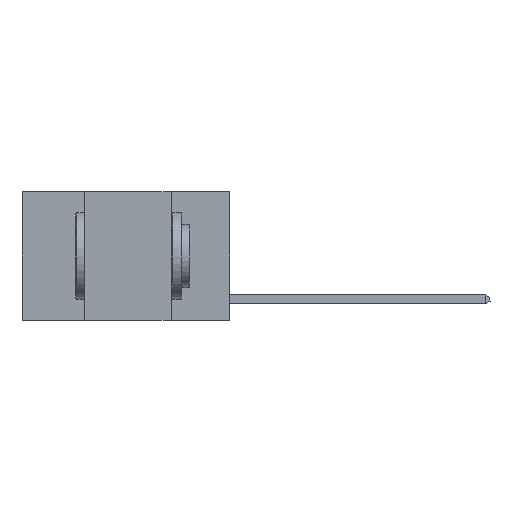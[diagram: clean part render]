
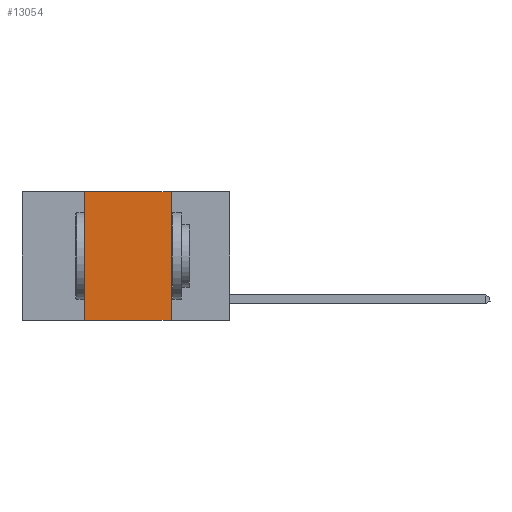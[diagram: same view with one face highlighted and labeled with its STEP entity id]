
A CAD part, left-side view. The second image highlights one B-rep face of the part: STEP entity #13054.
In plain terms, the highlighted planar face has unit normal (-1, 0, 0).
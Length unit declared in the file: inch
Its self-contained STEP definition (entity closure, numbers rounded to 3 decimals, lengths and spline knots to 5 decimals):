
#703 = VERTEX_POINT ( 'NONE', #8760 ) ;
#841 = VECTOR ( 'NONE', #3938, 39.37008 ) ;
#972 = VERTEX_POINT ( 'NONE', #12482 ) ;
#1309 = ORIENTED_EDGE ( 'NONE', *, *, #9274, .F. ) ;
#1996 = ORIENTED_EDGE ( 'NONE', *, *, #3330, .T. ) ;
#2269 = CARTESIAN_POINT ( 'NONE',  ( 0., 0.6, 0. ) ) ;
#2640 = VECTOR ( 'NONE', #10468, 39.37008 ) ;
#2839 = CARTESIAN_POINT ( 'NONE',  ( 0., 0.17, 0. ) ) ;
#3330 = EDGE_CURVE ( 'NONE', #8530, #703, #12839, .T. ) ;
#3938 = DIRECTION ( 'NONE',  ( 0., 0., -1. ) ) ;
#4167 = CARTESIAN_POINT ( 'NONE',  ( 0., 0.42, 0. ) ) ;
#4551 = LINE ( 'NONE', #2839, #841 ) ;
#4772 = PLANE ( 'NONE',  #9886 ) ;
#4812 = CARTESIAN_POINT ( 'NONE',  ( 0., 0.42, -0.37 ) ) ;
#5056 = EDGE_CURVE ( 'NONE', #8530, #972, #5558, .T. ) ;
#5394 = CARTESIAN_POINT ( 'NONE',  ( 0., 0.17, 0. ) ) ;
#5558 = LINE ( 'NONE', #4167, #2640 ) ;
#6608 = DIRECTION ( 'NONE',  ( 0., -1., 0. ) ) ;
#6929 = DIRECTION ( 'NONE',  ( 0., 0., -1. ) ) ;
#7650 = EDGE_CURVE ( 'NONE', #972, #11025, #9418, .T. ) ;
#8530 = VERTEX_POINT ( 'NONE', #4812 ) ;
#8760 = CARTESIAN_POINT ( 'NONE',  ( 0., 0.17, -0.37 ) ) ;
#9109 = VECTOR ( 'NONE', #6608, 39.37008 ) ;
#9274 = EDGE_CURVE ( 'NONE', #11025, #703, #4551, .T. ) ;
#9418 = LINE ( 'NONE', #2269, #9109 ) ;
#9662 = CARTESIAN_POINT ( 'NONE',  ( 0., 0.6, -0.37 ) ) ;
#9886 = AXIS2_PLACEMENT_3D ( 'NONE', #12046, #13043, #6929 ) ;
#10434 = EDGE_LOOP ( 'NONE', ( #1309, #12005, #10498, #1996 ) ) ;
#10468 = DIRECTION ( 'NONE',  ( 0., 0., 1. ) ) ;
#10498 = ORIENTED_EDGE ( 'NONE', *, *, #5056, .F. ) ;
#11025 = VERTEX_POINT ( 'NONE', #5394 ) ;
#12005 = ORIENTED_EDGE ( 'NONE', *, *, #7650, .F. ) ;
#12046 = CARTESIAN_POINT ( 'NONE',  ( 0., 0.6, 0. ) ) ;
#12482 = CARTESIAN_POINT ( 'NONE',  ( 0., 0.42, 0. ) ) ;
#12522 = VECTOR ( 'NONE', #12734, 39.37008 ) ;
#12734 = DIRECTION ( 'NONE',  ( 0., -1., 0. ) ) ;
#12839 = LINE ( 'NONE', #9662, #12522 ) ;
#13043 = DIRECTION ( 'NONE',  ( 1., 0., 0. ) ) ;
#13054 = ADVANCED_FACE ( 'NONE', ( #13194 ), #4772, .F. ) ;
#13194 = FACE_OUTER_BOUND ( 'NONE', #10434, .T. ) ;
